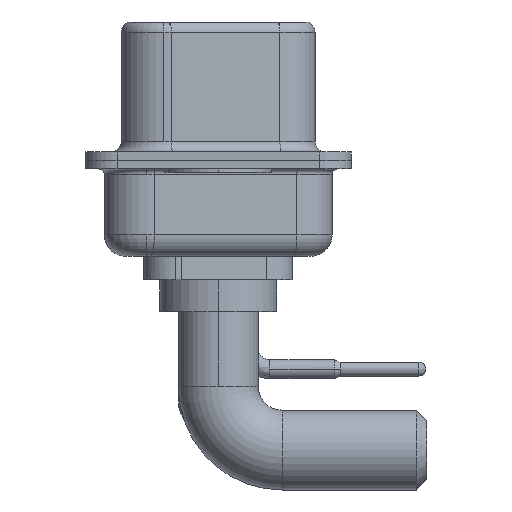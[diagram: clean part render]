
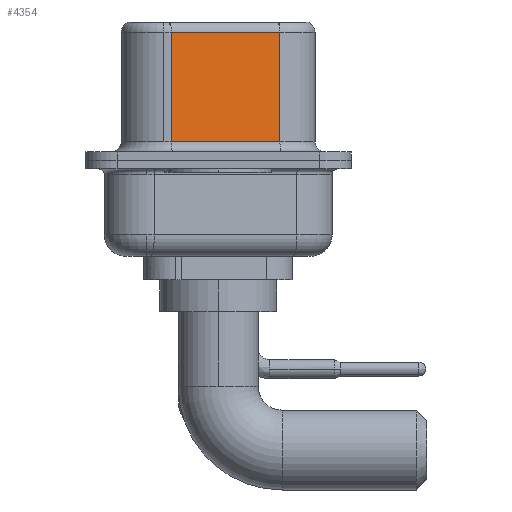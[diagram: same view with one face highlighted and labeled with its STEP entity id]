
A CAD part, left-side view. The second image highlights one B-rep face of the part: STEP entity #4354.
In plain terms, the highlighted planar face has unit normal (-0.985, -0.174, 0).
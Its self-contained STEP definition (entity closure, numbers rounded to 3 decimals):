
#538 = CARTESIAN_POINT ( 'NONE',  ( 4.58, -2.897, 6.52 ) ) ;
#1291 = DIRECTION ( 'NONE',  ( 0.174, -0.985, 0. ) ) ;
#1771 = EDGE_CURVE ( 'NONE', #6638, #18647, #25855, .T. ) ;
#2338 = ORIENTED_EDGE ( 'NONE', *, *, #23415, .F. ) ;
#4235 = CARTESIAN_POINT ( 'NONE',  ( 4.58, -2.897, 6.02 ) ) ;
#4354 = ADVANCED_FACE ( 'NONE', ( #18646 ), #20248, .F. ) ;
#4718 = DIRECTION ( 'NONE',  ( 0., 0., -1. ) ) ;
#5294 = ORIENTED_EDGE ( 'NONE', *, *, #1771, .T. ) ;
#5712 = ORIENTED_EDGE ( 'NONE', *, *, #18393, .T. ) ;
#6482 = DIRECTION ( 'NONE',  ( -0.174, 0.985, 0. ) ) ;
#6638 = VERTEX_POINT ( 'NONE', #13793 ) ;
#7530 = VECTOR ( 'NONE', #23461, 1000. ) ;
#7732 = LINE ( 'NONE', #22007, #7530 ) ;
#9718 = VECTOR ( 'NONE', #1291, 1000. ) ;
#11703 = CARTESIAN_POINT ( 'NONE',  ( 4.58, -2.897, 0.9 ) ) ;
#12710 = EDGE_CURVE ( 'NONE', #22508, #18373, #7732, .T. ) ;
#13793 = CARTESIAN_POINT ( 'NONE',  ( 3.68, 2.203, 0.9 ) ) ;
#14731 = EDGE_LOOP ( 'NONE', ( #2338, #23015, #5712, #5294 ) ) ;
#15155 = CARTESIAN_POINT ( 'NONE',  ( 4.58, -2.897, 6.52 ) ) ;
#16642 = DIRECTION ( 'NONE',  ( 0.985, 0.174, 0. ) ) ;
#17084 = VECTOR ( 'NONE', #25081, 1000. ) ;
#18373 = VERTEX_POINT ( 'NONE', #21653 ) ;
#18393 = EDGE_CURVE ( 'NONE', #18373, #6638, #20325, .T. ) ;
#18646 = FACE_OUTER_BOUND ( 'NONE', #14731, .T. ) ;
#18647 = VERTEX_POINT ( 'NONE', #24950 ) ;
#20219 = VECTOR ( 'NONE', #4718, 1000. ) ;
#20248 = PLANE ( 'NONE',  #24450 ) ;
#20325 = LINE ( 'NONE', #20579, #20219 ) ;
#20579 = CARTESIAN_POINT ( 'NONE',  ( 3.68, 2.203, 6.52 ) ) ;
#21653 = CARTESIAN_POINT ( 'NONE',  ( 3.68, 2.203, 6.02 ) ) ;
#22007 = CARTESIAN_POINT ( 'NONE',  ( 4.58, -2.897, 6.02 ) ) ;
#22508 = VERTEX_POINT ( 'NONE', #4235 ) ;
#22953 = LINE ( 'NONE', #15155, #17084 ) ;
#23015 = ORIENTED_EDGE ( 'NONE', *, *, #12710, .T. ) ;
#23415 = EDGE_CURVE ( 'NONE', #22508, #18647, #22953, .T. ) ;
#23461 = DIRECTION ( 'NONE',  ( -0.174, 0.985, 0. ) ) ;
#24450 = AXIS2_PLACEMENT_3D ( 'NONE', #538, #16642, #6482 ) ;
#24950 = CARTESIAN_POINT ( 'NONE',  ( 4.58, -2.897, 0.9 ) ) ;
#25081 = DIRECTION ( 'NONE',  ( 0., 0., -1. ) ) ;
#25855 = LINE ( 'NONE', #11703, #9718 ) ;
